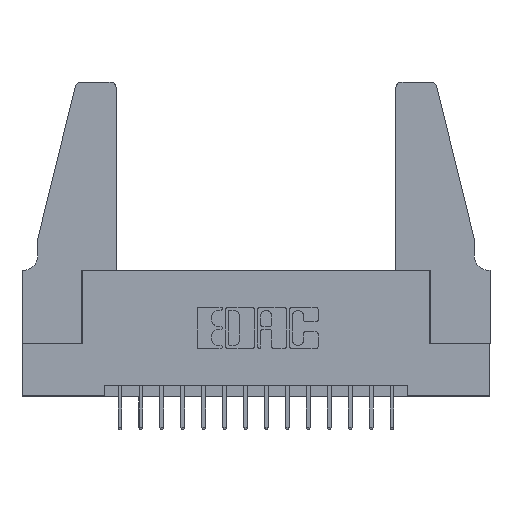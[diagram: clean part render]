
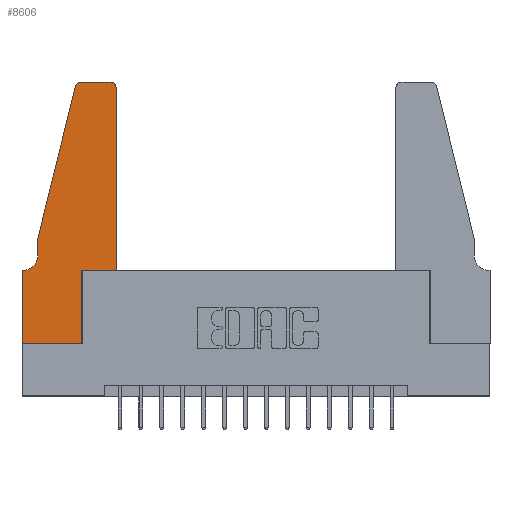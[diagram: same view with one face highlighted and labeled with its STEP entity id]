
A CAD part, top view. The second image highlights one B-rep face of the part: STEP entity #8606.
In plain terms, the highlighted planar face has unit normal (0, 0, 1).
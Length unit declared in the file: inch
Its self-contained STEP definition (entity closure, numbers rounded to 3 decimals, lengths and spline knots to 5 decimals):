
#254 = DIRECTION ( 'NONE',  ( 0., 1., 0. ) ) ;
#324 = CARTESIAN_POINT ( 'NONE',  ( 0.4505, 0.35, 0.37 ) ) ;
#339 = CARTESIAN_POINT ( 'NONE',  ( 0.4505, 0.35, 0.37 ) ) ;
#342 = VECTOR ( 'NONE', #3633, 39.37008 ) ;
#370 = ORIENTED_EDGE ( 'NONE', *, *, #3113, .T. ) ;
#648 = LINE ( 'NONE', #14703, #14319 ) ;
#653 = CARTESIAN_POINT ( 'NONE',  ( 0.0755, 0.35, 0.37 ) ) ;
#747 = EDGE_CURVE ( 'NONE', #7338, #12239, #9126, .T. ) ;
#776 = EDGE_CURVE ( 'NONE', #13539, #3629, #1567, .T. ) ;
#1134 = DIRECTION ( 'NONE',  ( 0., 0., -1. ) ) ;
#1379 = LINE ( 'NONE', #2206, #14948 ) ;
#1552 = CARTESIAN_POINT ( 'NONE',  ( 0.0755, 0.42, 0.37 ) ) ;
#1567 = LINE ( 'NONE', #5913, #15115 ) ;
#1808 = VERTEX_POINT ( 'NONE', #9854 ) ;
#1938 = ORIENTED_EDGE ( 'NONE', *, *, #13183, .T. ) ;
#1946 = CARTESIAN_POINT ( 'NONE',  ( 0.4505, 0.35, 0.37 ) ) ;
#1996 = VECTOR ( 'NONE', #2108, 39.37008 ) ;
#2079 = LINE ( 'NONE', #653, #15574 ) ;
#2093 = DIRECTION ( 'NONE',  ( -1., 0., 0. ) ) ;
#2108 = DIRECTION ( 'NONE',  ( 0., 1., 0. ) ) ;
#2206 = CARTESIAN_POINT ( 'NONE',  ( 0., 0., 0.37 ) ) ;
#2286 = VERTEX_POINT ( 'NONE', #15538 ) ;
#2374 = ORIENTED_EDGE ( 'NONE', *, *, #776, .T. ) ;
#2704 = VECTOR ( 'NONE', #5254, 39.37008 ) ;
#2784 = ORIENTED_EDGE ( 'NONE', *, *, #4763, .T. ) ;
#2955 = EDGE_CURVE ( 'NONE', #8153, #7338, #14052, .T. ) ;
#3031 = DIRECTION ( 'NONE',  ( -0.239, -0.971, 0. ) ) ;
#3113 = EDGE_CURVE ( 'NONE', #16000, #6412, #12843, .T. ) ;
#3222 = ORIENTED_EDGE ( 'NONE', *, *, #2955, .T. ) ;
#3320 = CARTESIAN_POINT ( 'NONE',  ( 0., 0.35, 0.37 ) ) ;
#3629 = VERTEX_POINT ( 'NONE', #1552 ) ;
#3633 = DIRECTION ( 'NONE',  ( 1., 0., 0. ) ) ;
#3636 = CARTESIAN_POINT ( 'NONE',  ( 0., 0., 0.37 ) ) ;
#3662 = ORIENTED_EDGE ( 'NONE', *, *, #5216, .T. ) ;
#3787 = CARTESIAN_POINT ( 'NONE',  ( 0.4205, 1.22, 0.37 ) ) ;
#4105 = ORIENTED_EDGE ( 'NONE', *, *, #4206, .T. ) ;
#4206 = EDGE_CURVE ( 'NONE', #6412, #1808, #13420, .T. ) ;
#4214 = VERTEX_POINT ( 'NONE', #6427 ) ;
#4476 = EDGE_LOOP ( 'NONE', ( #1938, #5591, #15833, #2374, #5998, #2784, #16583, #3222, #16954, #3662, #370, #4105 ) ) ;
#4721 = PLANE ( 'NONE',  #6189 ) ;
#4763 = EDGE_CURVE ( 'NONE', #2286, #12152, #2079, .T. ) ;
#4764 = CARTESIAN_POINT ( 'NONE',  ( 0.2865, 0., 0.37 ) ) ;
#4987 = DIRECTION ( 'NONE',  ( 0., -1., 0. ) ) ;
#5180 = DIRECTION ( 'NONE',  ( 1., 0., 0. ) ) ;
#5216 = EDGE_CURVE ( 'NONE', #12239, #16000, #16309, .T. ) ;
#5254 = DIRECTION ( 'NONE',  ( -1., 0., 0. ) ) ;
#5377 = CIRCLE ( 'NONE', #16471, 0.07 ) ;
#5591 = ORIENTED_EDGE ( 'NONE', *, *, #13157, .T. ) ;
#5913 = CARTESIAN_POINT ( 'NONE',  ( 0.0755, 0.5, 0.37 ) ) ;
#5998 = ORIENTED_EDGE ( 'NONE', *, *, #8869, .T. ) ;
#6050 = DIRECTION ( 'NONE',  ( 0., 0., 1. ) ) ;
#6189 = AXIS2_PLACEMENT_3D ( 'NONE', #3320, #6050, #15058 ) ;
#6412 = VERTEX_POINT ( 'NONE', #14864 ) ;
#6427 = CARTESIAN_POINT ( 'NONE',  ( 0.25487, 1.22718, 0.37 ) ) ;
#6642 = EDGE_CURVE ( 'NONE', #12152, #8153, #1379, .T. ) ;
#6699 = AXIS2_PLACEMENT_3D ( 'NONE', #3787, #12932, #5180 ) ;
#7338 = VERTEX_POINT ( 'NONE', #4764 ) ;
#7564 = CARTESIAN_POINT ( 'NONE',  ( 0.2865, 0.35, 0.37 ) ) ;
#7823 = EDGE_CURVE ( 'NONE', #4214, #13539, #648, .T. ) ;
#7856 = DIRECTION ( 'NONE',  ( 0., 0., 1. ) ) ;
#8153 = VERTEX_POINT ( 'NONE', #14193 ) ;
#8166 = CARTESIAN_POINT ( 'NONE',  ( 0.2865, 0.35, 0.37 ) ) ;
#8572 = CARTESIAN_POINT ( 'NONE',  ( 0.0755, 0.5, 0.37 ) ) ;
#8606 = ADVANCED_FACE ( 'NONE', ( #16221 ), #4721, .T. ) ;
#8869 = EDGE_CURVE ( 'NONE', #3629, #2286, #5377, .T. ) ;
#9126 = LINE ( 'NONE', #8166, #1996 ) ;
#9147 = CARTESIAN_POINT ( 'NONE',  ( 0.2605, 1.25, 0.37 ) ) ;
#9193 = CARTESIAN_POINT ( 'NONE',  ( 0.0055, 0.42, 0.37 ) ) ;
#9212 = VERTEX_POINT ( 'NONE', #9839 ) ;
#9839 = CARTESIAN_POINT ( 'NONE',  ( 0.284, 1.25, 0.37 ) ) ;
#9854 = CARTESIAN_POINT ( 'NONE',  ( 0.4205, 1.25, 0.37 ) ) ;
#10464 = DIRECTION ( 'NONE',  ( -1., 0., 0. ) ) ;
#11053 = AXIS2_PLACEMENT_3D ( 'NONE', #15502, #7856, #16707 ) ;
#11261 = CARTESIAN_POINT ( 'NONE',  ( 0., 0.35, 0.37 ) ) ;
#12152 = VERTEX_POINT ( 'NONE', #11261 ) ;
#12239 = VERTEX_POINT ( 'NONE', #7564 ) ;
#12433 = DIRECTION ( 'NONE',  ( 1., 0., 0. ) ) ;
#12795 = CIRCLE ( 'NONE', #11053, 0.03 ) ;
#12843 = LINE ( 'NONE', #339, #15435 ) ;
#12932 = DIRECTION ( 'NONE',  ( 0., 0., 1. ) ) ;
#13157 = EDGE_CURVE ( 'NONE', #9212, #4214, #12795, .T. ) ;
#13183 = EDGE_CURVE ( 'NONE', #1808, #9212, #15765, .T. ) ;
#13420 = CIRCLE ( 'NONE', #6699, 0.03 ) ;
#13539 = VERTEX_POINT ( 'NONE', #8572 ) ;
#14052 = LINE ( 'NONE', #3636, #342 ) ;
#14193 = CARTESIAN_POINT ( 'NONE',  ( 0., 0., 0.37 ) ) ;
#14319 = VECTOR ( 'NONE', #3031, 39.37008 ) ;
#14478 = DIRECTION ( 'NONE',  ( 0., -1., 0. ) ) ;
#14703 = CARTESIAN_POINT ( 'NONE',  ( 0.0755, 0.5, 0.37 ) ) ;
#14864 = CARTESIAN_POINT ( 'NONE',  ( 0.4505, 1.22, 0.37 ) ) ;
#14948 = VECTOR ( 'NONE', #4987, 39.37008 ) ;
#15058 = DIRECTION ( 'NONE',  ( 1., 0., 0. ) ) ;
#15115 = VECTOR ( 'NONE', #14478, 39.37008 ) ;
#15435 = VECTOR ( 'NONE', #254, 39.37008 ) ;
#15502 = CARTESIAN_POINT ( 'NONE',  ( 0.284, 1.22, 0.37 ) ) ;
#15538 = CARTESIAN_POINT ( 'NONE',  ( 0.0055, 0.35, 0.37 ) ) ;
#15574 = VECTOR ( 'NONE', #2093, 39.37008 ) ;
#15765 = LINE ( 'NONE', #9147, #2704 ) ;
#15833 = ORIENTED_EDGE ( 'NONE', *, *, #7823, .T. ) ;
#15939 = VECTOR ( 'NONE', #12433, 39.37008 ) ;
#16000 = VERTEX_POINT ( 'NONE', #324 ) ;
#16221 = FACE_OUTER_BOUND ( 'NONE', #4476, .T. ) ;
#16309 = LINE ( 'NONE', #1946, #15939 ) ;
#16471 = AXIS2_PLACEMENT_3D ( 'NONE', #9193, #1134, #10464 ) ;
#16583 = ORIENTED_EDGE ( 'NONE', *, *, #6642, .T. ) ;
#16707 = DIRECTION ( 'NONE',  ( 1., 0., 0. ) ) ;
#16954 = ORIENTED_EDGE ( 'NONE', *, *, #747, .T. ) ;
